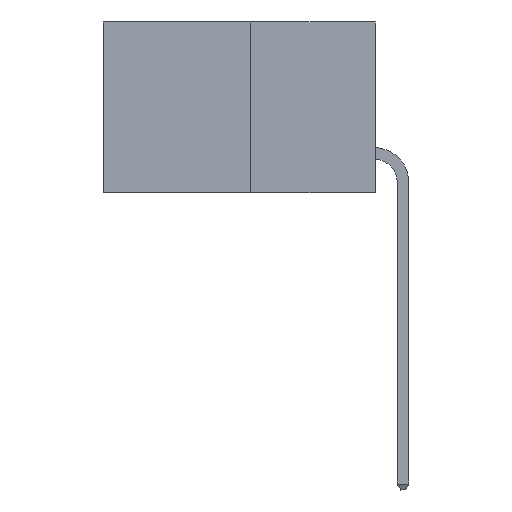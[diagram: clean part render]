
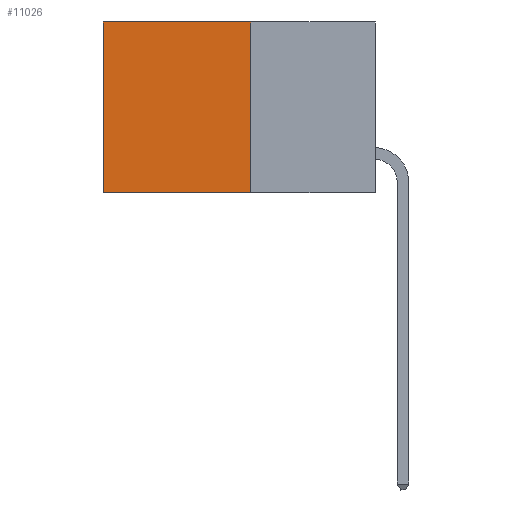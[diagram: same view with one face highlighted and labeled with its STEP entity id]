
A CAD part, left-side view. The second image highlights one B-rep face of the part: STEP entity #11026.
In plain terms, the highlighted planar face has unit normal (-1, 0, 0).
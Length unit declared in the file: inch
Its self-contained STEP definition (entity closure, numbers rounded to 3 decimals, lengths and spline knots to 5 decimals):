
#854 = EDGE_CURVE ( 'NONE', #10477, #4303, #10665, .T. ) ;
#1696 = EDGE_CURVE ( 'NONE', #10477, #5454, #12198, .T. ) ;
#2016 = VERTEX_POINT ( 'NONE', #7866 ) ;
#2329 = CARTESIAN_POINT ( 'NONE',  ( 0.277, 0.27, -0.37 ) ) ;
#2501 = DIRECTION ( 'NONE',  ( 0., 0., -1. ) ) ;
#3059 = EDGE_CURVE ( 'NONE', #5454, #2016, #8955, .T. ) ;
#3266 = CARTESIAN_POINT ( 'NONE',  ( 0.277, 0.27, 0. ) ) ;
#3321 = VECTOR ( 'NONE', #5871, 39.37008 ) ;
#3425 = ORIENTED_EDGE ( 'NONE', *, *, #3059, .T. ) ;
#4067 = EDGE_CURVE ( 'NONE', #4303, #2016, #8200, .T. ) ;
#4303 = VERTEX_POINT ( 'NONE', #4346 ) ;
#4346 = CARTESIAN_POINT ( 'NONE',  ( 0.277, 0.27, -0.37 ) ) ;
#4778 = VECTOR ( 'NONE', #5180, 39.37008 ) ;
#5180 = DIRECTION ( 'NONE',  ( 0., 1., 0. ) ) ;
#5454 = VERTEX_POINT ( 'NONE', #11371 ) ;
#5608 = AXIS2_PLACEMENT_3D ( 'NONE', #12008, #8444, #2501 ) ;
#5663 = VECTOR ( 'NONE', #6326, 39.37008 ) ;
#5871 = DIRECTION ( 'NONE',  ( 0., 0., -1. ) ) ;
#6094 = ORIENTED_EDGE ( 'NONE', *, *, #4067, .F. ) ;
#6319 = CARTESIAN_POINT ( 'NONE',  ( 0.277, 0.27, -0.37 ) ) ;
#6326 = DIRECTION ( 'NONE',  ( 0., 1., 0. ) ) ;
#6388 = ORIENTED_EDGE ( 'NONE', *, *, #854, .F. ) ;
#7866 = CARTESIAN_POINT ( 'NONE',  ( 0.277, 0.59, -0.37 ) ) ;
#8200 = LINE ( 'NONE', #6319, #5663 ) ;
#8403 = PLANE ( 'NONE',  #5608 ) ;
#8444 = DIRECTION ( 'NONE',  ( 1., 0., 0. ) ) ;
#8672 = VECTOR ( 'NONE', #9413, 39.37008 ) ;
#8894 = ORIENTED_EDGE ( 'NONE', *, *, #1696, .T. ) ;
#8955 = LINE ( 'NONE', #9894, #8672 ) ;
#9105 = FACE_OUTER_BOUND ( 'NONE', #10180, .T. ) ;
#9413 = DIRECTION ( 'NONE',  ( 0., 0., -1. ) ) ;
#9894 = CARTESIAN_POINT ( 'NONE',  ( 0.277, 0.59, -0.37 ) ) ;
#10180 = EDGE_LOOP ( 'NONE', ( #3425, #6094, #6388, #8894 ) ) ;
#10477 = VERTEX_POINT ( 'NONE', #11287 ) ;
#10665 = LINE ( 'NONE', #2329, #3321 ) ;
#11026 = ADVANCED_FACE ( 'NONE', ( #9105 ), #8403, .F. ) ;
#11287 = CARTESIAN_POINT ( 'NONE',  ( 0.277, 0.27, 0. ) ) ;
#11371 = CARTESIAN_POINT ( 'NONE',  ( 0.277, 0.59, 0. ) ) ;
#12008 = CARTESIAN_POINT ( 'NONE',  ( 0.277, 0.27, -0.37 ) ) ;
#12198 = LINE ( 'NONE', #3266, #4778 ) ;
